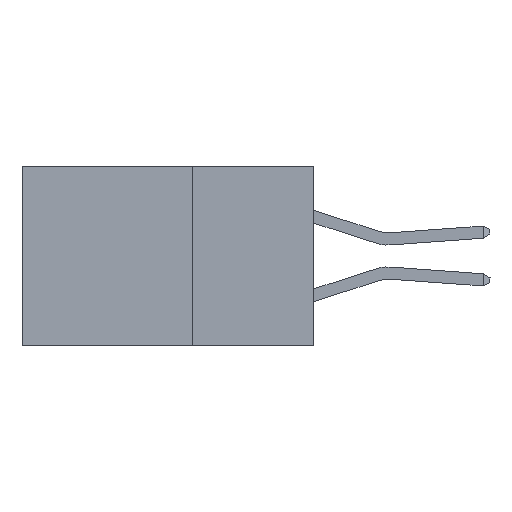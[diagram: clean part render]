
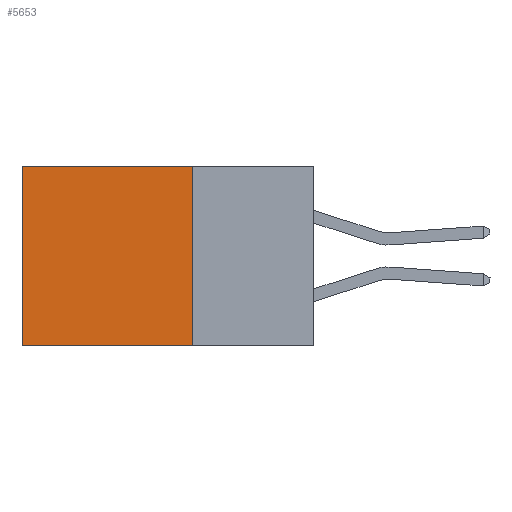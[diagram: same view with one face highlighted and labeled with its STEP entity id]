
A CAD part, left-side view. The second image highlights one B-rep face of the part: STEP entity #5653.
In plain terms, the highlighted planar face has unit normal (-1, 0, 0).
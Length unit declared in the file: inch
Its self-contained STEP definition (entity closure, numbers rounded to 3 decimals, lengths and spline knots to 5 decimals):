
#455 = EDGE_CURVE ( 'NONE', #6049, #12747, #10436, .T. ) ;
#507 = EDGE_CURVE ( 'NONE', #6049, #12432, #8602, .T. ) ;
#862 = CARTESIAN_POINT ( 'NONE',  ( 0.2875, 0.25, 0. ) ) ;
#1551 = EDGE_CURVE ( 'NONE', #12747, #10409, #4284, .T. ) ;
#1990 = ORIENTED_EDGE ( 'NONE', *, *, #1551, .T. ) ;
#2042 = VECTOR ( 'NONE', #6872, 39.37008 ) ;
#2151 = EDGE_LOOP ( 'NONE', ( #1990, #7020, #9078, #10480 ) ) ;
#2383 = VECTOR ( 'NONE', #4804, 39.37008 ) ;
#2614 = CARTESIAN_POINT ( 'NONE',  ( 0.2875, 0.25, -0.37 ) ) ;
#3700 = EDGE_CURVE ( 'NONE', #12432, #10409, #8280, .T. ) ;
#3794 = DIRECTION ( 'NONE',  ( 0., 0., -1. ) ) ;
#4154 = CARTESIAN_POINT ( 'NONE',  ( 0.2875, 0.6, 0. ) ) ;
#4284 = LINE ( 'NONE', #10775, #8805 ) ;
#4750 = DIRECTION ( 'NONE',  ( 1., 0., 0. ) ) ;
#4804 = DIRECTION ( 'NONE',  ( 0., 1., 0. ) ) ;
#4860 = CARTESIAN_POINT ( 'NONE',  ( 0.2875, 0.25, -0.37 ) ) ;
#5653 = ADVANCED_FACE ( 'NONE', ( #13225 ), #9749, .F. ) ;
#6049 = VERTEX_POINT ( 'NONE', #862 ) ;
#6052 = CARTESIAN_POINT ( 'NONE',  ( 0.2875, 0.25, 0. ) ) ;
#6482 = VECTOR ( 'NONE', #3794, 39.37008 ) ;
#6872 = DIRECTION ( 'NONE',  ( 0., 1., 0. ) ) ;
#7020 = ORIENTED_EDGE ( 'NONE', *, *, #3700, .F. ) ;
#8280 = LINE ( 'NONE', #4860, #2383 ) ;
#8602 = LINE ( 'NONE', #6052, #6482 ) ;
#8805 = VECTOR ( 'NONE', #9549, 39.37008 ) ;
#9078 = ORIENTED_EDGE ( 'NONE', *, *, #507, .F. ) ;
#9160 = CARTESIAN_POINT ( 'NONE',  ( 0.2875, 0.6, -0.37 ) ) ;
#9549 = DIRECTION ( 'NONE',  ( 0., 0., -1. ) ) ;
#9749 = PLANE ( 'NONE',  #10189 ) ;
#10189 = AXIS2_PLACEMENT_3D ( 'NONE', #11512, #4750, #11548 ) ;
#10409 = VERTEX_POINT ( 'NONE', #9160 ) ;
#10436 = LINE ( 'NONE', #11087, #2042 ) ;
#10480 = ORIENTED_EDGE ( 'NONE', *, *, #455, .T. ) ;
#10775 = CARTESIAN_POINT ( 'NONE',  ( 0.2875, 0.6, 0. ) ) ;
#11087 = CARTESIAN_POINT ( 'NONE',  ( 0.2875, 0.25, 0. ) ) ;
#11512 = CARTESIAN_POINT ( 'NONE',  ( 0.2875, 0.25, 0. ) ) ;
#11548 = DIRECTION ( 'NONE',  ( 0., 0., -1. ) ) ;
#12432 = VERTEX_POINT ( 'NONE', #2614 ) ;
#12747 = VERTEX_POINT ( 'NONE', #4154 ) ;
#13225 = FACE_OUTER_BOUND ( 'NONE', #2151, .T. ) ;
